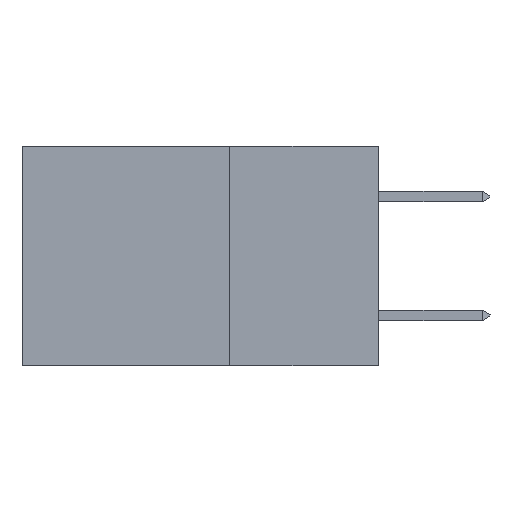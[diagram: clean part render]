
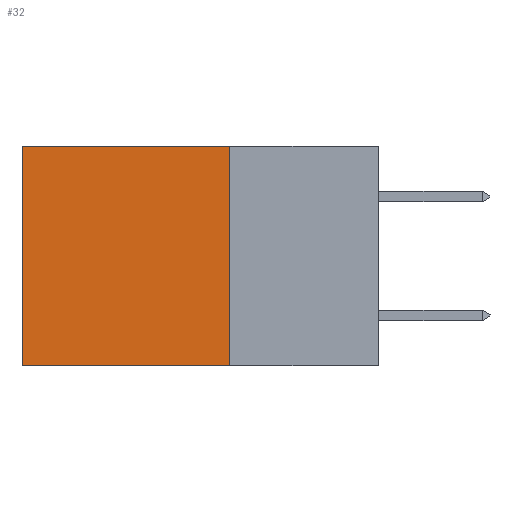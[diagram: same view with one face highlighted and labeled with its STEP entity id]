
A CAD part, left-side view. The second image highlights one B-rep face of the part: STEP entity #32.
In plain terms, the highlighted planar face has unit normal (-1, 0, 0).
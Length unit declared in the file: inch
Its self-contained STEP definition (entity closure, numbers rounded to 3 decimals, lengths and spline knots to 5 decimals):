
#32 = ADVANCED_FACE ( 'NONE', ( #8468 ), #1691, .F. ) ;
#253 = DIRECTION ( 'NONE',  ( 0., 0., -1. ) ) ;
#1691 = PLANE ( 'NONE',  #12487 ) ;
#2030 = CARTESIAN_POINT ( 'NONE',  ( 0.298, 0.25, 0. ) ) ;
#2100 = EDGE_LOOP ( 'NONE', ( #12853, #20760, #22253, #2899 ) ) ;
#2815 = CARTESIAN_POINT ( 'NONE',  ( 0.298, 0.6, -0.37 ) ) ;
#2899 = ORIENTED_EDGE ( 'NONE', *, *, #18749, .T. ) ;
#3085 = LINE ( 'NONE', #14383, #13019 ) ;
#4297 = VERTEX_POINT ( 'NONE', #2815 ) ;
#5001 = DIRECTION ( 'NONE',  ( 1., 0., 0. ) ) ;
#5198 = CARTESIAN_POINT ( 'NONE',  ( 0.298, 0.25, -0.37 ) ) ;
#5931 = EDGE_CURVE ( 'NONE', #12255, #4297, #3085, .T. ) ;
#6839 = VECTOR ( 'NONE', #9002, 39.37008 ) ;
#7028 = VERTEX_POINT ( 'NONE', #19924 ) ;
#7038 = VERTEX_POINT ( 'NONE', #8263 ) ;
#7243 = EDGE_CURVE ( 'NONE', #7038, #4297, #18037, .T. ) ;
#7647 = DIRECTION ( 'NONE',  ( 0., 0., -1. ) ) ;
#7921 = LINE ( 'NONE', #2030, #6839 ) ;
#8263 = CARTESIAN_POINT ( 'NONE',  ( 0.298, 0.25, -0.37 ) ) ;
#8468 = FACE_OUTER_BOUND ( 'NONE', #2100, .T. ) ;
#8617 = CARTESIAN_POINT ( 'NONE',  ( 0.298, 0.25, 0. ) ) ;
#9002 = DIRECTION ( 'NONE',  ( 0., 1., 0. ) ) ;
#9155 = LINE ( 'NONE', #8617, #16938 ) ;
#10315 = CARTESIAN_POINT ( 'NONE',  ( 0.298, 0.25, 0. ) ) ;
#10355 = DIRECTION ( 'NONE',  ( 0., 1., 0. ) ) ;
#12255 = VERTEX_POINT ( 'NONE', #20229 ) ;
#12487 = AXIS2_PLACEMENT_3D ( 'NONE', #10315, #5001, #18734 ) ;
#12853 = ORIENTED_EDGE ( 'NONE', *, *, #5931, .T. ) ;
#13019 = VECTOR ( 'NONE', #7647, 39.37008 ) ;
#14292 = EDGE_CURVE ( 'NONE', #7028, #7038, #9155, .T. ) ;
#14383 = CARTESIAN_POINT ( 'NONE',  ( 0.298, 0.6, 0. ) ) ;
#16938 = VECTOR ( 'NONE', #253, 39.37008 ) ;
#17495 = VECTOR ( 'NONE', #10355, 39.37008 ) ;
#18037 = LINE ( 'NONE', #5198, #17495 ) ;
#18734 = DIRECTION ( 'NONE',  ( 0., 0., -1. ) ) ;
#18749 = EDGE_CURVE ( 'NONE', #7028, #12255, #7921, .T. ) ;
#19924 = CARTESIAN_POINT ( 'NONE',  ( 0.298, 0.25, 0. ) ) ;
#20229 = CARTESIAN_POINT ( 'NONE',  ( 0.298, 0.6, 0. ) ) ;
#20760 = ORIENTED_EDGE ( 'NONE', *, *, #7243, .F. ) ;
#22253 = ORIENTED_EDGE ( 'NONE', *, *, #14292, .F. ) ;
